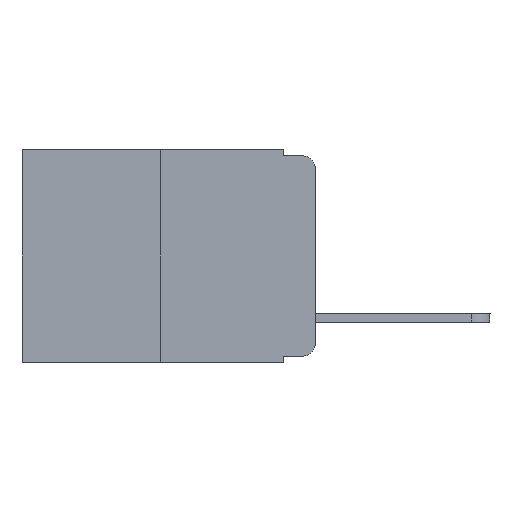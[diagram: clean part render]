
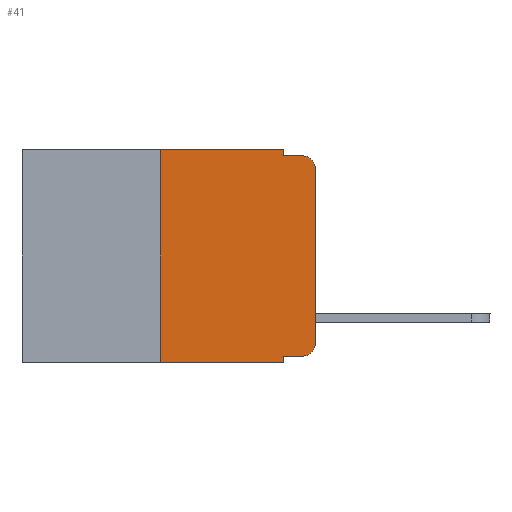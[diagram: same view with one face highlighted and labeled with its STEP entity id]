
A CAD part, left-side view. The second image highlights one B-rep face of the part: STEP entity #41.
In plain terms, the highlighted planar face has unit normal (-1, 0, 0).
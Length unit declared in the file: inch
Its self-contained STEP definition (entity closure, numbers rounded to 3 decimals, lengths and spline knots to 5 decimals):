
#41 = ADVANCED_FACE ( 'NONE', ( #1298 ), #305, .F. ) ;
#163 = CARTESIAN_POINT ( 'NONE',  ( 0., 0.473, 0. ) ) ;
#186 = LINE ( 'NONE', #12564, #7230 ) ;
#305 = PLANE ( 'NONE',  #5098 ) ;
#515 = LINE ( 'NONE', #12689, #11927 ) ;
#544 = ORIENTED_EDGE ( 'NONE', *, *, #11706, .F. ) ;
#582 = CARTESIAN_POINT ( 'NONE',  ( 0., 0.051, -0.333 ) ) ;
#743 = VERTEX_POINT ( 'NONE', #1415 ) ;
#1089 = VECTOR ( 'NONE', #1825, 39.37008 ) ;
#1224 = ORIENTED_EDGE ( 'NONE', *, *, #7149, .F. ) ;
#1249 = CARTESIAN_POINT ( 'NONE',  ( 0., 0.051, -0.343 ) ) ;
#1298 = FACE_OUTER_BOUND ( 'NONE', #10658, .T. ) ;
#1415 = CARTESIAN_POINT ( 'NONE',  ( 0., 0.02, -0.333 ) ) ;
#1648 = VERTEX_POINT ( 'NONE', #6358 ) ;
#1738 = ORIENTED_EDGE ( 'NONE', *, *, #2200, .T. ) ;
#1825 = DIRECTION ( 'NONE',  ( 0., -1., 0. ) ) ;
#1963 = CARTESIAN_POINT ( 'NONE',  ( 0., 0.473, -0.343 ) ) ;
#2001 = DIRECTION ( 'NONE',  ( -1., 0., 0. ) ) ;
#2018 = CARTESIAN_POINT ( 'NONE',  ( 0., 0.051, -0.01 ) ) ;
#2200 = EDGE_CURVE ( 'NONE', #8469, #9761, #6138, .T. ) ;
#2391 = ORIENTED_EDGE ( 'NONE', *, *, #9922, .T. ) ;
#2772 = DIRECTION ( 'NONE',  ( 0., 0., 1. ) ) ;
#2827 = LINE ( 'NONE', #1963, #1089 ) ;
#2837 = EDGE_CURVE ( 'NONE', #10856, #743, #6362, .T. ) ;
#2838 = VECTOR ( 'NONE', #3962, 39.37008 ) ;
#2840 = EDGE_CURVE ( 'NONE', #10856, #5180, #515, .T. ) ;
#3037 = AXIS2_PLACEMENT_3D ( 'NONE', #11148, #2001, #6039 ) ;
#3263 = DIRECTION ( 'NONE',  ( 0., 0., -1. ) ) ;
#3645 = LINE ( 'NONE', #6961, #13059 ) ;
#3962 = DIRECTION ( 'NONE',  ( 0., 0., 1. ) ) ;
#3978 = DIRECTION ( 'NONE',  ( 0., -1., 0. ) ) ;
#4184 = DIRECTION ( 'NONE',  ( 0., 0., -1. ) ) ;
#4225 = DIRECTION ( 'NONE',  ( 1., 0., 0. ) ) ;
#4263 = CARTESIAN_POINT ( 'NONE',  ( 0., 0.02, -0.03 ) ) ;
#4384 = DIRECTION ( 'NONE',  ( 0., -1., 0. ) ) ;
#4472 = AXIS2_PLACEMENT_3D ( 'NONE', #4263, #12320, #9282 ) ;
#4646 = EDGE_CURVE ( 'NONE', #11326, #8469, #4945, .T. ) ;
#4854 = CARTESIAN_POINT ( 'NONE',  ( 0., 0.051, -0.01 ) ) ;
#4881 = VECTOR ( 'NONE', #3978, 39.37008 ) ;
#4938 = VERTEX_POINT ( 'NONE', #4854 ) ;
#4945 = LINE ( 'NONE', #9014, #2838 ) ;
#5041 = ORIENTED_EDGE ( 'NONE', *, *, #7773, .F. ) ;
#5098 = AXIS2_PLACEMENT_3D ( 'NONE', #163, #4225, #3263 ) ;
#5180 = VERTEX_POINT ( 'NONE', #1249 ) ;
#5656 = ORIENTED_EDGE ( 'NONE', *, *, #7605, .F. ) ;
#5835 = CARTESIAN_POINT ( 'NONE',  ( 0., 0., -0.03 ) ) ;
#6039 = DIRECTION ( 'NONE',  ( 0., 0., -1. ) ) ;
#6092 = VERTEX_POINT ( 'NONE', #10359 ) ;
#6138 = CIRCLE ( 'NONE', #4472, 0.02 ) ;
#6358 = CARTESIAN_POINT ( 'NONE',  ( 0., 0.051, 0. ) ) ;
#6362 = LINE ( 'NONE', #582, #11693 ) ;
#6829 = CARTESIAN_POINT ( 'NONE',  ( 0., 0., -0.313 ) ) ;
#6961 = CARTESIAN_POINT ( 'NONE',  ( 0., 0.25, 0. ) ) ;
#7149 = EDGE_CURVE ( 'NONE', #6092, #1648, #7828, .T. ) ;
#7230 = VECTOR ( 'NONE', #4184, 39.37008 ) ;
#7508 = DIRECTION ( 'NONE',  ( 0., 0., -1. ) ) ;
#7605 = EDGE_CURVE ( 'NONE', #4938, #9761, #11034, .T. ) ;
#7723 = VERTEX_POINT ( 'NONE', #11355 ) ;
#7773 = EDGE_CURVE ( 'NONE', #1648, #4938, #186, .T. ) ;
#7828 = LINE ( 'NONE', #9033, #4881 ) ;
#8469 = VERTEX_POINT ( 'NONE', #5835 ) ;
#9004 = DIRECTION ( 'NONE',  ( 0., -1., 0. ) ) ;
#9014 = CARTESIAN_POINT ( 'NONE',  ( 0., 0., 0. ) ) ;
#9033 = CARTESIAN_POINT ( 'NONE',  ( 0., 0.473, 0. ) ) ;
#9282 = DIRECTION ( 'NONE',  ( 0., 0., -1. ) ) ;
#9451 = VECTOR ( 'NONE', #9004, 39.37008 ) ;
#9761 = VERTEX_POINT ( 'NONE', #10885 ) ;
#9922 = EDGE_CURVE ( 'NONE', #743, #11326, #10698, .T. ) ;
#10147 = ORIENTED_EDGE ( 'NONE', *, *, #2840, .F. ) ;
#10359 = CARTESIAN_POINT ( 'NONE',  ( 0., 0.25, 0. ) ) ;
#10567 = EDGE_CURVE ( 'NONE', #7723, #5180, #2827, .T. ) ;
#10658 = EDGE_LOOP ( 'NONE', ( #11274, #1738, #5656, #5041, #1224, #544, #11657, #10147, #12126, #2391 ) ) ;
#10698 = CIRCLE ( 'NONE', #3037, 0.02 ) ;
#10856 = VERTEX_POINT ( 'NONE', #12839 ) ;
#10885 = CARTESIAN_POINT ( 'NONE',  ( 0., 0.02, -0.01 ) ) ;
#11034 = LINE ( 'NONE', #2018, #9451 ) ;
#11148 = CARTESIAN_POINT ( 'NONE',  ( 0., 0.02, -0.313 ) ) ;
#11274 = ORIENTED_EDGE ( 'NONE', *, *, #4646, .T. ) ;
#11326 = VERTEX_POINT ( 'NONE', #6829 ) ;
#11355 = CARTESIAN_POINT ( 'NONE',  ( 0., 0.25, -0.343 ) ) ;
#11657 = ORIENTED_EDGE ( 'NONE', *, *, #10567, .T. ) ;
#11693 = VECTOR ( 'NONE', #4384, 39.37008 ) ;
#11706 = EDGE_CURVE ( 'NONE', #7723, #6092, #3645, .T. ) ;
#11927 = VECTOR ( 'NONE', #7508, 39.37008 ) ;
#12126 = ORIENTED_EDGE ( 'NONE', *, *, #2837, .T. ) ;
#12320 = DIRECTION ( 'NONE',  ( -1., 0., 0. ) ) ;
#12564 = CARTESIAN_POINT ( 'NONE',  ( 0., 0.051, 0. ) ) ;
#12689 = CARTESIAN_POINT ( 'NONE',  ( 0., 0.051, 0. ) ) ;
#12839 = CARTESIAN_POINT ( 'NONE',  ( 0., 0.051, -0.333 ) ) ;
#13059 = VECTOR ( 'NONE', #2772, 39.37008 ) ;
